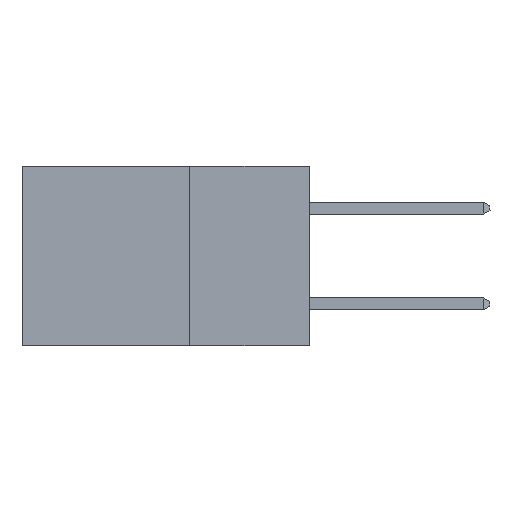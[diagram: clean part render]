
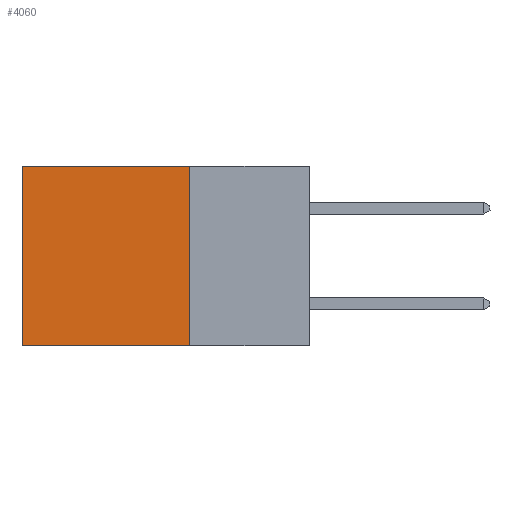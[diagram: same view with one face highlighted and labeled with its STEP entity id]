
A CAD part, left-side view. The second image highlights one B-rep face of the part: STEP entity #4060.
In plain terms, the highlighted planar face has unit normal (-1, 0, 0).
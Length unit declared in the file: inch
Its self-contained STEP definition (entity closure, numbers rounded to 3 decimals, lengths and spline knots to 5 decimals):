
#2 = VECTOR ( 'NONE', #631, 39.37008 ) ;
#455 = CARTESIAN_POINT ( 'NONE',  ( 0.2875, 0.25, 0. ) ) ;
#631 = DIRECTION ( 'NONE',  ( 0., 0., -1. ) ) ;
#1265 = CARTESIAN_POINT ( 'NONE',  ( 0.2875, 0.6, -0.375 ) ) ;
#1650 = ORIENTED_EDGE ( 'NONE', *, *, #8243, .F. ) ;
#1943 = ORIENTED_EDGE ( 'NONE', *, *, #6784, .T. ) ;
#1985 = FACE_OUTER_BOUND ( 'NONE', #4996, .T. ) ;
#2480 = VECTOR ( 'NONE', #5653, 39.37008 ) ;
#2734 = AXIS2_PLACEMENT_3D ( 'NONE', #6508, #7327, #6452 ) ;
#3185 = CARTESIAN_POINT ( 'NONE',  ( 0.2875, 0.6, -0.375 ) ) ;
#3194 = ORIENTED_EDGE ( 'NONE', *, *, #8516, .F. ) ;
#3336 = VERTEX_POINT ( 'NONE', #8048 ) ;
#3511 = CARTESIAN_POINT ( 'NONE',  ( 0.2875, 0.25, -0.375 ) ) ;
#3687 = ORIENTED_EDGE ( 'NONE', *, *, #9200, .T. ) ;
#4060 = ADVANCED_FACE ( 'NONE', ( #1985 ), #9463, .F. ) ;
#4528 = CARTESIAN_POINT ( 'NONE',  ( 0.2875, 0.25, -0.375 ) ) ;
#4543 = VERTEX_POINT ( 'NONE', #3185 ) ;
#4553 = CARTESIAN_POINT ( 'NONE',  ( 0.2875, 0.25, -0.375 ) ) ;
#4946 = DIRECTION ( 'NONE',  ( 0., 1., 0. ) ) ;
#4996 = EDGE_LOOP ( 'NONE', ( #3687, #3194, #1650, #1943 ) ) ;
#5052 = CARTESIAN_POINT ( 'NONE',  ( 0.2875, 0.25, 0. ) ) ;
#5653 = DIRECTION ( 'NONE',  ( 0., 1., 0. ) ) ;
#5672 = LINE ( 'NONE', #5052, #5788 ) ;
#5788 = VECTOR ( 'NONE', #4946, 39.37008 ) ;
#6452 = DIRECTION ( 'NONE',  ( 0., 0., -1. ) ) ;
#6480 = LINE ( 'NONE', #3511, #2480 ) ;
#6508 = CARTESIAN_POINT ( 'NONE',  ( 0.2875, 0.25, -0.375 ) ) ;
#6784 = EDGE_CURVE ( 'NONE', #7312, #3336, #5672, .T. ) ;
#6977 = VECTOR ( 'NONE', #7581, 39.37008 ) ;
#7073 = LINE ( 'NONE', #1265, #2 ) ;
#7312 = VERTEX_POINT ( 'NONE', #455 ) ;
#7327 = DIRECTION ( 'NONE',  ( 1., 0., 0. ) ) ;
#7562 = LINE ( 'NONE', #4528, #6977 ) ;
#7581 = DIRECTION ( 'NONE',  ( 0., 0., -1. ) ) ;
#8048 = CARTESIAN_POINT ( 'NONE',  ( 0.2875, 0.6, 0. ) ) ;
#8243 = EDGE_CURVE ( 'NONE', #7312, #8805, #7562, .T. ) ;
#8516 = EDGE_CURVE ( 'NONE', #8805, #4543, #6480, .T. ) ;
#8805 = VERTEX_POINT ( 'NONE', #4553 ) ;
#9200 = EDGE_CURVE ( 'NONE', #3336, #4543, #7073, .T. ) ;
#9463 = PLANE ( 'NONE',  #2734 ) ;
